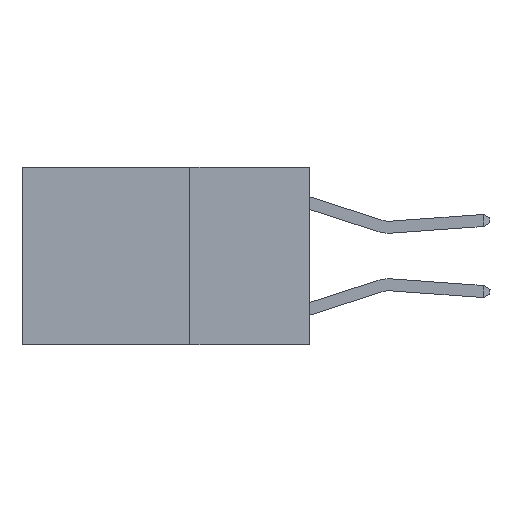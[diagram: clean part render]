
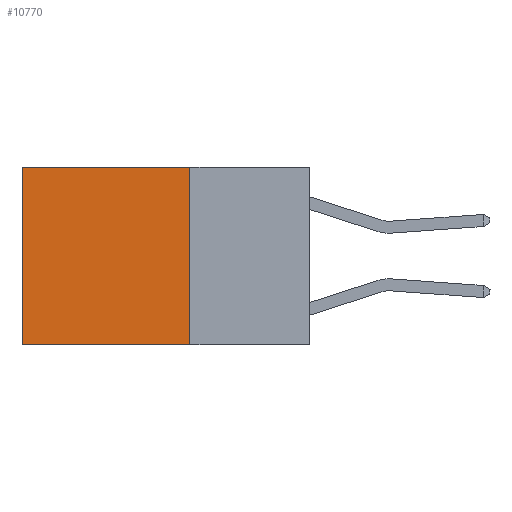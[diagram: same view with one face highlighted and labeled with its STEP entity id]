
A CAD part, left-side view. The second image highlights one B-rep face of the part: STEP entity #10770.
In plain terms, the highlighted planar face has unit normal (-1, 0, 0).
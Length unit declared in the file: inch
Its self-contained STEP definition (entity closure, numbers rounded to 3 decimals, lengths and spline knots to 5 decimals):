
#1665 = ORIENTED_EDGE ( 'NONE', *, *, #2590, .T. ) ;
#2590 = EDGE_CURVE ( 'NONE', #5706, #28051, #11175, .T. ) ;
#3793 = ORIENTED_EDGE ( 'NONE', *, *, #24031, .T. ) ;
#4148 = VECTOR ( 'NONE', #16884, 39.37008 ) ;
#4246 = VECTOR ( 'NONE', #23408, 39.37008 ) ;
#4993 = LINE ( 'NONE', #16452, #4246 ) ;
#5024 = CARTESIAN_POINT ( 'NONE',  ( 0.2625, 0.6, -0.37 ) ) ;
#5706 = VERTEX_POINT ( 'NONE', #26560 ) ;
#8041 = LINE ( 'NONE', #16095, #20658 ) ;
#10696 = PLANE ( 'NONE',  #24210 ) ;
#10770 = ADVANCED_FACE ( 'NONE', ( #11098 ), #10696, .F. ) ;
#11098 = FACE_OUTER_BOUND ( 'NONE', #22565, .T. ) ;
#11175 = LINE ( 'NONE', #23168, #16682 ) ;
#12425 = EDGE_CURVE ( 'NONE', #5706, #15406, #16873, .T. ) ;
#14545 = CARTESIAN_POINT ( 'NONE',  ( 0.2625, 0.25, 0. ) ) ;
#14790 = CARTESIAN_POINT ( 'NONE',  ( 0.2625, 0.25, -0.37 ) ) ;
#15406 = VERTEX_POINT ( 'NONE', #14790 ) ;
#15444 = DIRECTION ( 'NONE',  ( 0., 0., -1. ) ) ;
#16095 = CARTESIAN_POINT ( 'NONE',  ( 0.2625, 0.25, -0.37 ) ) ;
#16452 = CARTESIAN_POINT ( 'NONE',  ( 0.2625, 0.6, 0. ) ) ;
#16682 = VECTOR ( 'NONE', #25498, 39.37008 ) ;
#16873 = LINE ( 'NONE', #14545, #4148 ) ;
#16884 = DIRECTION ( 'NONE',  ( 0., 0., -1. ) ) ;
#18264 = EDGE_CURVE ( 'NONE', #15406, #19261, #8041, .T. ) ;
#19261 = VERTEX_POINT ( 'NONE', #5024 ) ;
#20656 = ORIENTED_EDGE ( 'NONE', *, *, #18264, .F. ) ;
#20658 = VECTOR ( 'NONE', #30074, 39.37008 ) ;
#22410 = CARTESIAN_POINT ( 'NONE',  ( 0.2625, 0.25, 0. ) ) ;
#22565 = EDGE_LOOP ( 'NONE', ( #3793, #20656, #23959, #1665 ) ) ;
#23113 = CARTESIAN_POINT ( 'NONE',  ( 0.2625, 0.6, 0. ) ) ;
#23168 = CARTESIAN_POINT ( 'NONE',  ( 0.2625, 0.25, 0. ) ) ;
#23408 = DIRECTION ( 'NONE',  ( 0., 0., -1. ) ) ;
#23959 = ORIENTED_EDGE ( 'NONE', *, *, #12425, .F. ) ;
#24031 = EDGE_CURVE ( 'NONE', #28051, #19261, #4993, .T. ) ;
#24210 = AXIS2_PLACEMENT_3D ( 'NONE', #22410, #29406, #15444 ) ;
#25498 = DIRECTION ( 'NONE',  ( 0., 1., 0. ) ) ;
#26560 = CARTESIAN_POINT ( 'NONE',  ( 0.2625, 0.25, 0. ) ) ;
#28051 = VERTEX_POINT ( 'NONE', #23113 ) ;
#29406 = DIRECTION ( 'NONE',  ( 1., 0., 0. ) ) ;
#30074 = DIRECTION ( 'NONE',  ( 0., 1., 0. ) ) ;
